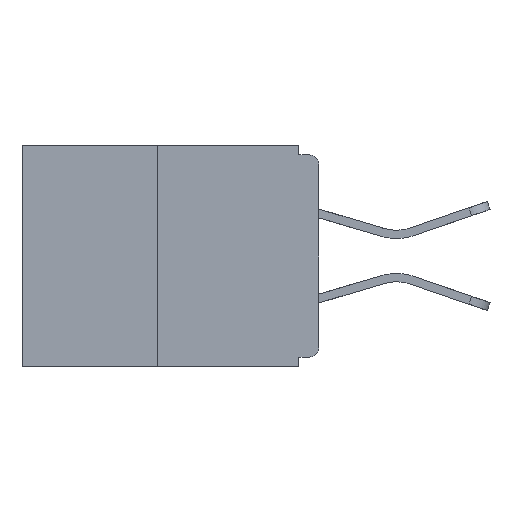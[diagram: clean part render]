
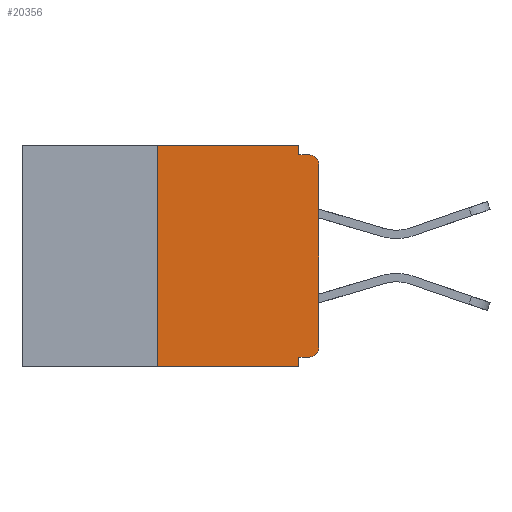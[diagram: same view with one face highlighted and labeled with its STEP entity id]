
A CAD part, left-side view. The second image highlights one B-rep face of the part: STEP entity #20356.
In plain terms, the highlighted planar face has unit normal (-1, 0, 0).
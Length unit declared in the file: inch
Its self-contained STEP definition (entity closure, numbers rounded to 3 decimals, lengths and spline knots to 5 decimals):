
#269 = ORIENTED_EDGE ( 'NONE', *, *, #1227, .T. ) ;
#408 = VECTOR ( 'NONE', #17300, 39.37008 ) ;
#475 = DIRECTION ( 'NONE',  ( 1., 0., 0. ) ) ;
#1153 = CARTESIAN_POINT ( 'NONE',  ( 0., 0.25, 0. ) ) ;
#1200 = DIRECTION ( 'NONE',  ( -1., 0., 0. ) ) ;
#1227 = EDGE_CURVE ( 'NONE', #19188, #16719, #2958, .T. ) ;
#1474 = CIRCLE ( 'NONE', #12420, 0.015 ) ;
#2265 = DIRECTION ( 'NONE',  ( 0., 0., -1. ) ) ;
#2287 = EDGE_CURVE ( 'NONE', #17770, #6532, #18896, .T. ) ;
#2374 = VECTOR ( 'NONE', #9503, 39.37008 ) ;
#2409 = ORIENTED_EDGE ( 'NONE', *, *, #18456, .F. ) ;
#2421 = VECTOR ( 'NONE', #19873, 39.37008 ) ;
#2958 = LINE ( 'NONE', #11454, #2421 ) ;
#3199 = LINE ( 'NONE', #17127, #19687 ) ;
#3315 = CARTESIAN_POINT ( 'NONE',  ( 0., 0.25, 0. ) ) ;
#3393 = CARTESIAN_POINT ( 'NONE',  ( 0., 0., -0.03 ) ) ;
#3504 = CARTESIAN_POINT ( 'NONE',  ( 0., 0.031, -0.343 ) ) ;
#3968 = AXIS2_PLACEMENT_3D ( 'NONE', #13896, #13963, #18744 ) ;
#4179 = EDGE_CURVE ( 'NONE', #16719, #6660, #1474, .T. ) ;
#4345 = VERTEX_POINT ( 'NONE', #18263 ) ;
#4377 = CARTESIAN_POINT ( 'NONE',  ( 0., 0.46, -0.343 ) ) ;
#4443 = ORIENTED_EDGE ( 'NONE', *, *, #14499, .F. ) ;
#4883 = CARTESIAN_POINT ( 'NONE',  ( 0., 0., -0.015 ) ) ;
#4929 = LINE ( 'NONE', #8937, #408 ) ;
#5145 = EDGE_CURVE ( 'NONE', #7294, #6532, #4929, .T. ) ;
#5154 = CARTESIAN_POINT ( 'NONE',  ( 0., 0., -0.328 ) ) ;
#5889 = LINE ( 'NONE', #19042, #8299 ) ;
#5918 = FACE_OUTER_BOUND ( 'NONE', #17974, .T. ) ;
#6007 = AXIS2_PLACEMENT_3D ( 'NONE', #17458, #475, #2265 ) ;
#6532 = VERTEX_POINT ( 'NONE', #3504 ) ;
#6660 = VERTEX_POINT ( 'NONE', #12398 ) ;
#7138 = CARTESIAN_POINT ( 'NONE',  ( 0., 0., -0.313 ) ) ;
#7294 = VERTEX_POINT ( 'NONE', #10482 ) ;
#7325 = VECTOR ( 'NONE', #12011, 39.37008 ) ;
#7333 = EDGE_CURVE ( 'NONE', #18277, #4345, #3199, .T. ) ;
#7726 = VERTEX_POINT ( 'NONE', #16270 ) ;
#8299 = VECTOR ( 'NONE', #14265, 39.37008 ) ;
#8937 = CARTESIAN_POINT ( 'NONE',  ( 0., 0.031, -0.343 ) ) ;
#9503 = DIRECTION ( 'NONE',  ( 0., -1., 0. ) ) ;
#10109 = ORIENTED_EDGE ( 'NONE', *, *, #5145, .F. ) ;
#10191 = VECTOR ( 'NONE', #13554, 39.37008 ) ;
#10333 = DIRECTION ( 'NONE',  ( 0., -1., 0. ) ) ;
#10482 = CARTESIAN_POINT ( 'NONE',  ( 0., 0.031, -0.328 ) ) ;
#11454 = CARTESIAN_POINT ( 'NONE',  ( 0., 0., 0. ) ) ;
#11615 = ORIENTED_EDGE ( 'NONE', *, *, #16243, .T. ) ;
#12011 = DIRECTION ( 'NONE',  ( 0., 1., 0. ) ) ;
#12221 = ORIENTED_EDGE ( 'NONE', *, *, #2287, .T. ) ;
#12398 = CARTESIAN_POINT ( 'NONE',  ( 0., 0.015, -0.015 ) ) ;
#12420 = AXIS2_PLACEMENT_3D ( 'NONE', #18256, #1200, #19879 ) ;
#12482 = ORIENTED_EDGE ( 'NONE', *, *, #14672, .F. ) ;
#12520 = PLANE ( 'NONE',  #6007 ) ;
#13001 = VERTEX_POINT ( 'NONE', #13931 ) ;
#13554 = DIRECTION ( 'NONE',  ( 0., 0., 1. ) ) ;
#13896 = CARTESIAN_POINT ( 'NONE',  ( 0., 0.015, -0.313 ) ) ;
#13931 = CARTESIAN_POINT ( 'NONE',  ( 0., 0.031, -0.015 ) ) ;
#13963 = DIRECTION ( 'NONE',  ( -1., 0., 0. ) ) ;
#14265 = DIRECTION ( 'NONE',  ( 0., 0., -1. ) ) ;
#14499 = EDGE_CURVE ( 'NONE', #17770, #18277, #15785, .T. ) ;
#14672 = EDGE_CURVE ( 'NONE', #4345, #13001, #5889, .T. ) ;
#15631 = VECTOR ( 'NONE', #16732, 39.37008 ) ;
#15785 = LINE ( 'NONE', #3315, #10191 ) ;
#15887 = ORIENTED_EDGE ( 'NONE', *, *, #7333, .F. ) ;
#16243 = EDGE_CURVE ( 'NONE', #7726, #19188, #20208, .T. ) ;
#16270 = CARTESIAN_POINT ( 'NONE',  ( 0., 0.015, -0.328 ) ) ;
#16694 = ORIENTED_EDGE ( 'NONE', *, *, #4179, .T. ) ;
#16719 = VERTEX_POINT ( 'NONE', #3393 ) ;
#16732 = DIRECTION ( 'NONE',  ( 0., -1., 0. ) ) ;
#17127 = CARTESIAN_POINT ( 'NONE',  ( 0., 0.46, 0. ) ) ;
#17300 = DIRECTION ( 'NONE',  ( 0., 0., -1. ) ) ;
#17458 = CARTESIAN_POINT ( 'NONE',  ( 0., 0.46, 0. ) ) ;
#17569 = EDGE_CURVE ( 'NONE', #13001, #6660, #22026, .T. ) ;
#17770 = VERTEX_POINT ( 'NONE', #21301 ) ;
#17967 = LINE ( 'NONE', #5154, #7325 ) ;
#17974 = EDGE_LOOP ( 'NONE', ( #15887, #4443, #12221, #10109, #2409, #11615, #269, #16694, #20066, #12482 ) ) ;
#18256 = CARTESIAN_POINT ( 'NONE',  ( 0., 0.015, -0.03 ) ) ;
#18263 = CARTESIAN_POINT ( 'NONE',  ( 0., 0.031, 0. ) ) ;
#18277 = VERTEX_POINT ( 'NONE', #1153 ) ;
#18456 = EDGE_CURVE ( 'NONE', #7726, #7294, #17967, .T. ) ;
#18744 = DIRECTION ( 'NONE',  ( 0., 0., -1. ) ) ;
#18896 = LINE ( 'NONE', #4377, #2374 ) ;
#19042 = CARTESIAN_POINT ( 'NONE',  ( 0., 0.031, 0. ) ) ;
#19188 = VERTEX_POINT ( 'NONE', #7138 ) ;
#19687 = VECTOR ( 'NONE', #10333, 39.37008 ) ;
#19873 = DIRECTION ( 'NONE',  ( 0., 0., 1. ) ) ;
#19879 = DIRECTION ( 'NONE',  ( 0., 0., -1. ) ) ;
#20066 = ORIENTED_EDGE ( 'NONE', *, *, #17569, .F. ) ;
#20208 = CIRCLE ( 'NONE', #3968, 0.015 ) ;
#20356 = ADVANCED_FACE ( 'NONE', ( #5918 ), #12520, .F. ) ;
#21301 = CARTESIAN_POINT ( 'NONE',  ( 0., 0.25, -0.343 ) ) ;
#22026 = LINE ( 'NONE', #4883, #15631 ) ;
